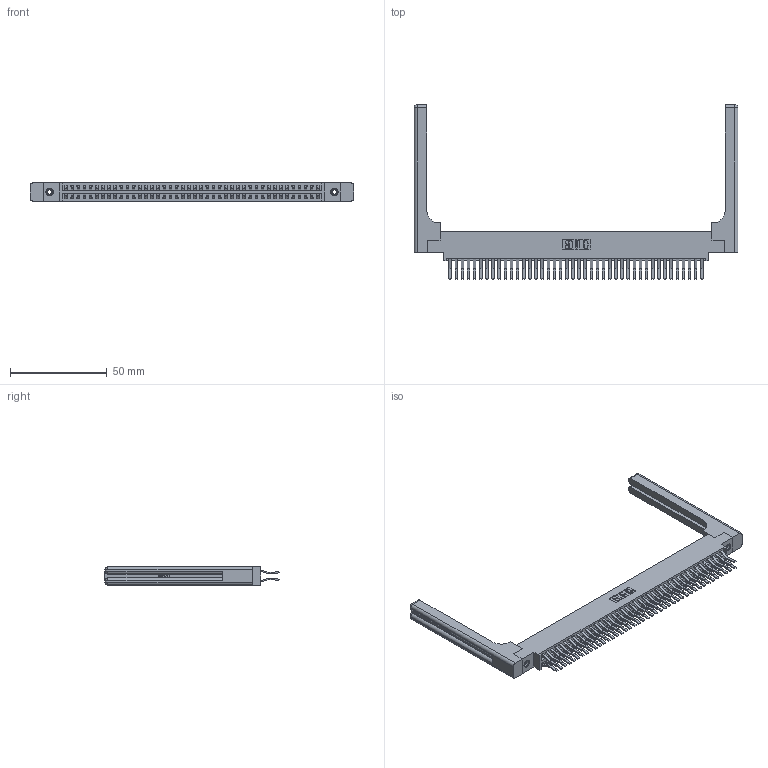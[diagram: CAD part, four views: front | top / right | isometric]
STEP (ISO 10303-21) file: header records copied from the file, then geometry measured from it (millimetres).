
FILE_DESCRIPTION (( 'STEP AP203' ), '1' );
FILE_NAME ('346-084-560-858.STEP', '2022-05-25T21:22:45', ( '' ), ( '' ), 'SwSTEP 2.0', 'SolidWorks 2020', '' );
FILE_SCHEMA (( 'CONFIG_CONTROL_DESIGN' ));
Length unit declared in the file: inch
Products named in the file (5): 345-292-001_560 Tail; 346 Part_0.170 Offset - 0.156 Dia-TH; 346-220-058_345-220-058; 345-250-001_345-250-001-102; 346-084-560-858
Assembly tree (89 placements, depth 2):
  346-084-560-858
    346 Part_0.170 Offset - 0.156 Dia-TH
    345-292-001_560 Tail  x84
    345-250-001_345-250-001-102  x2
    346-220-058_345-220-058  x2
Bounding box: 167.41 x 90.05 x 9.4 mm (x, y, z)
Volume: 24196.8 mm3; surface area: 29614.7 mm2
Topology: 89 solids, 89 shells, 4932 faces, 14567 edges, 9578 vertices
Faces by surface type: plane 3182, cylinder 1690, bspline 36, cone 12, sphere 8, torus 4
Entity records: 33228 total; most frequent: CARTESIAN_POINT 6491, ORIENTED_EDGE 5220, DIRECTION 4706, EDGE_CURVE 2610, LINE 2214, VECTOR 2214, VERTEX_POINT 1730, AXIS2_PLACEMENT_3D 1246
